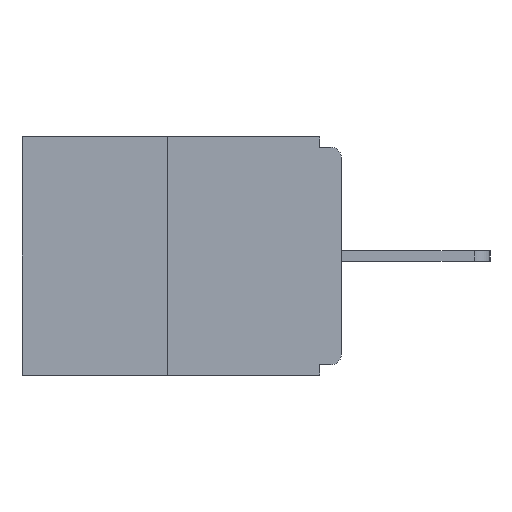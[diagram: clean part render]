
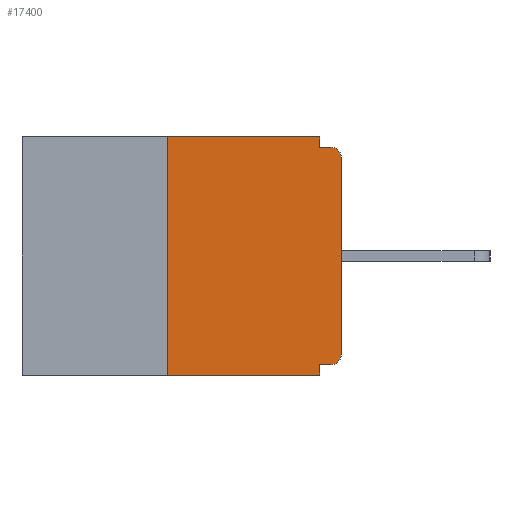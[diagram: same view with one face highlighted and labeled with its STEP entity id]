
A CAD part, left-side view. The second image highlights one B-rep face of the part: STEP entity #17400.
In plain terms, the highlighted planar face has unit normal (-1, 0, 0).
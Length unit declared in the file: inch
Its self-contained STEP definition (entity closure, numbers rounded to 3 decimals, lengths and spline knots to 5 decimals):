
#27 = DIRECTION ( 'NONE',  ( 1., 0., 0. ) ) ;
#88 = CARTESIAN_POINT ( 'NONE',  ( 0., 0.015, -0.015 ) ) ;
#183 = AXIS2_PLACEMENT_3D ( 'NONE', #8065, #27, #16452 ) ;
#624 = LINE ( 'NONE', #1977, #14250 ) ;
#1185 = VECTOR ( 'NONE', #13000, 39.37008 ) ;
#1371 = CARTESIAN_POINT ( 'NONE',  ( 0., 0.46, 0. ) ) ;
#1513 = EDGE_LOOP ( 'NONE', ( #6469, #3826, #14572, #10333, #3350, #14150, #10969, #14764, #12332, #1945 ) ) ;
#1616 = CARTESIAN_POINT ( 'NONE',  ( 0., 0.015, -0.03 ) ) ;
#1623 = EDGE_CURVE ( 'NONE', #14577, #14468, #5857, .T. ) ;
#1632 = EDGE_CURVE ( 'NONE', #11412, #7423, #4504, .T. ) ;
#1761 = LINE ( 'NONE', #4832, #4735 ) ;
#1945 = ORIENTED_EDGE ( 'NONE', *, *, #1632, .F. ) ;
#1977 = CARTESIAN_POINT ( 'NONE',  ( 0., 0.031, -0.343 ) ) ;
#2895 = CARTESIAN_POINT ( 'NONE',  ( 0., 0.031, -0.343 ) ) ;
#3350 = ORIENTED_EDGE ( 'NONE', *, *, #4957, .F. ) ;
#3535 = DIRECTION ( 'NONE',  ( 0., -1., 0. ) ) ;
#3826 = ORIENTED_EDGE ( 'NONE', *, *, #15214, .F. ) ;
#4058 = VECTOR ( 'NONE', #3535, 39.37008 ) ;
#4114 = LINE ( 'NONE', #12514, #14242 ) ;
#4321 = DIRECTION ( 'NONE',  ( 0., 0., -1. ) ) ;
#4504 = LINE ( 'NONE', #15515, #16509 ) ;
#4663 = EDGE_CURVE ( 'NONE', #13207, #8829, #4114, .T. ) ;
#4723 = VECTOR ( 'NONE', #14344, 39.37008 ) ;
#4735 = VECTOR ( 'NONE', #10343, 39.37008 ) ;
#4777 = DIRECTION ( 'NONE',  ( 0., 0., -1. ) ) ;
#4832 = CARTESIAN_POINT ( 'NONE',  ( 0., 0., -0.328 ) ) ;
#4957 = EDGE_CURVE ( 'NONE', #8230, #11697, #1761, .T. ) ;
#5164 = CIRCLE ( 'NONE', #15256, 0.015 ) ;
#5236 = LINE ( 'NONE', #17689, #16341 ) ;
#5256 = PLANE ( 'NONE',  #183 ) ;
#5754 = CARTESIAN_POINT ( 'NONE',  ( 0., 0.015, -0.328 ) ) ;
#5857 = LINE ( 'NONE', #6039, #4723 ) ;
#6039 = CARTESIAN_POINT ( 'NONE',  ( 0., 0., 0. ) ) ;
#6469 = ORIENTED_EDGE ( 'NONE', *, *, #11019, .F. ) ;
#7423 = VERTEX_POINT ( 'NONE', #14901 ) ;
#7899 = CARTESIAN_POINT ( 'NONE',  ( 0., 0., -0.03 ) ) ;
#8065 = CARTESIAN_POINT ( 'NONE',  ( 0., 0.46, 0. ) ) ;
#8230 = VERTEX_POINT ( 'NONE', #5754 ) ;
#8829 = VERTEX_POINT ( 'NONE', #2895 ) ;
#9106 = CARTESIAN_POINT ( 'NONE',  ( 0., 0.015, -0.313 ) ) ;
#9141 = EDGE_CURVE ( 'NONE', #8230, #14577, #5164, .T. ) ;
#10325 = CARTESIAN_POINT ( 'NONE',  ( 0., 0., -0.015 ) ) ;
#10333 = ORIENTED_EDGE ( 'NONE', *, *, #14099, .F. ) ;
#10343 = DIRECTION ( 'NONE',  ( 0., 1., 0. ) ) ;
#10677 = EDGE_CURVE ( 'NONE', #7423, #13951, #15899, .T. ) ;
#10969 = ORIENTED_EDGE ( 'NONE', *, *, #1623, .T. ) ;
#11019 = EDGE_CURVE ( 'NONE', #12238, #11412, #16443, .T. ) ;
#11027 = CARTESIAN_POINT ( 'NONE',  ( 0., 0.25, 0. ) ) ;
#11032 = FACE_OUTER_BOUND ( 'NONE', #1513, .T. ) ;
#11067 = DIRECTION ( 'NONE',  ( 0., -1., 0. ) ) ;
#11412 = VERTEX_POINT ( 'NONE', #15306 ) ;
#11565 = CARTESIAN_POINT ( 'NONE',  ( 0., 0., -0.313 ) ) ;
#11637 = DIRECTION ( 'NONE',  ( 0., 0., -1. ) ) ;
#11647 = CIRCLE ( 'NONE', #13949, 0.015 ) ;
#11697 = VERTEX_POINT ( 'NONE', #17727 ) ;
#11735 = DIRECTION ( 'NONE',  ( -1., 0., 0. ) ) ;
#12191 = DIRECTION ( 'NONE',  ( 0., 0., 1. ) ) ;
#12238 = VERTEX_POINT ( 'NONE', #11027 ) ;
#12332 = ORIENTED_EDGE ( 'NONE', *, *, #10677, .F. ) ;
#12514 = CARTESIAN_POINT ( 'NONE',  ( 0., 0.46, -0.343 ) ) ;
#12700 = CARTESIAN_POINT ( 'NONE',  ( 0., 0.25, -0.343 ) ) ;
#13000 = DIRECTION ( 'NONE',  ( 0., -1., 0. ) ) ;
#13207 = VERTEX_POINT ( 'NONE', #12700 ) ;
#13949 = AXIS2_PLACEMENT_3D ( 'NONE', #1616, #15599, #4777 ) ;
#13951 = VERTEX_POINT ( 'NONE', #88 ) ;
#14099 = EDGE_CURVE ( 'NONE', #11697, #8829, #624, .T. ) ;
#14150 = ORIENTED_EDGE ( 'NONE', *, *, #9141, .T. ) ;
#14242 = VECTOR ( 'NONE', #11067, 39.37008 ) ;
#14250 = VECTOR ( 'NONE', #11637, 39.37008 ) ;
#14344 = DIRECTION ( 'NONE',  ( 0., 0., 1. ) ) ;
#14468 = VERTEX_POINT ( 'NONE', #7899 ) ;
#14516 = DIRECTION ( 'NONE',  ( 0., 0., -1. ) ) ;
#14572 = ORIENTED_EDGE ( 'NONE', *, *, #4663, .T. ) ;
#14577 = VERTEX_POINT ( 'NONE', #11565 ) ;
#14764 = ORIENTED_EDGE ( 'NONE', *, *, #14992, .T. ) ;
#14901 = CARTESIAN_POINT ( 'NONE',  ( 0., 0.031, -0.015 ) ) ;
#14992 = EDGE_CURVE ( 'NONE', #14468, #13951, #11647, .T. ) ;
#15214 = EDGE_CURVE ( 'NONE', #13207, #12238, #5236, .T. ) ;
#15256 = AXIS2_PLACEMENT_3D ( 'NONE', #9106, #11735, #14516 ) ;
#15306 = CARTESIAN_POINT ( 'NONE',  ( 0., 0.031, 0. ) ) ;
#15515 = CARTESIAN_POINT ( 'NONE',  ( 0., 0.031, 0. ) ) ;
#15599 = DIRECTION ( 'NONE',  ( -1., 0., 0. ) ) ;
#15899 = LINE ( 'NONE', #10325, #4058 ) ;
#16341 = VECTOR ( 'NONE', #12191, 39.37008 ) ;
#16443 = LINE ( 'NONE', #1371, #1185 ) ;
#16452 = DIRECTION ( 'NONE',  ( 0., 0., -1. ) ) ;
#16509 = VECTOR ( 'NONE', #4321, 39.37008 ) ;
#17400 = ADVANCED_FACE ( 'NONE', ( #11032 ), #5256, .F. ) ;
#17689 = CARTESIAN_POINT ( 'NONE',  ( 0., 0.25, 0. ) ) ;
#17727 = CARTESIAN_POINT ( 'NONE',  ( 0., 0.031, -0.328 ) ) ;
